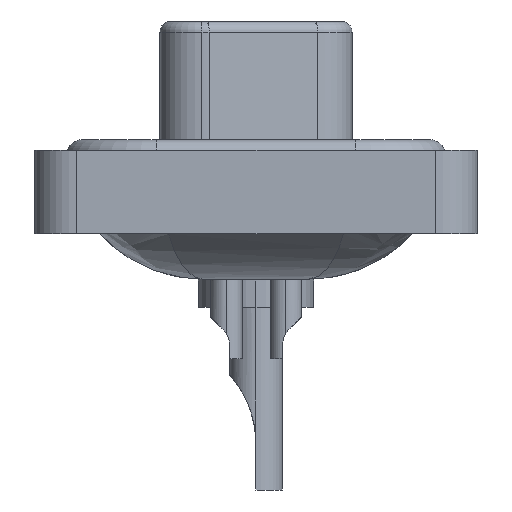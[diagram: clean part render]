
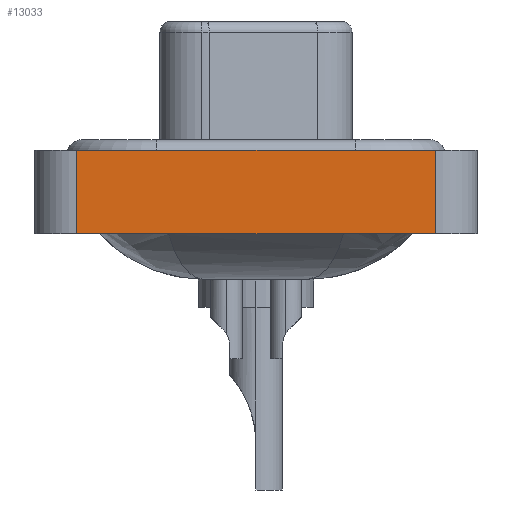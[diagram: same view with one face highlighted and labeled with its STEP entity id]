
A CAD part, left-side view. The second image highlights one B-rep face of the part: STEP entity #13033.
In plain terms, the highlighted planar face has unit normal (-1, 0, 0).
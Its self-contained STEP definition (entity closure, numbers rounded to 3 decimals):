
#166 = EDGE_CURVE ( 'NONE', #8085, #24075, #15353, .T. ) ;
#1186 = CARTESIAN_POINT ( 'NONE',  ( -7.35, 8.55, -3.6 ) ) ;
#1572 = VERTEX_POINT ( 'NONE', #1186 ) ;
#1585 = CARTESIAN_POINT ( 'NONE',  ( -7.35, 8.55, 0.4 ) ) ;
#3384 = DIRECTION ( 'NONE',  ( -1., 0., 0. ) ) ;
#3736 = DIRECTION ( 'NONE',  ( 0., 0., 1. ) ) ;
#4155 = LINE ( 'NONE', #21446, #20333 ) ;
#4780 = LINE ( 'NONE', #17997, #12625 ) ;
#5246 = FACE_OUTER_BOUND ( 'NONE', #16064, .T. ) ;
#5494 = CARTESIAN_POINT ( 'NONE',  ( -7.35, 8.55, -3.6 ) ) ;
#6149 = DIRECTION ( 'NONE',  ( 0., -1., 0. ) ) ;
#6770 = VERTEX_POINT ( 'NONE', #1585 ) ;
#8085 = VERTEX_POINT ( 'NONE', #16706 ) ;
#11334 = VECTOR ( 'NONE', #22654, 1000. ) ;
#11402 = CARTESIAN_POINT ( 'NONE',  ( -7.35, -8.55, -3.6 ) ) ;
#11580 = EDGE_CURVE ( 'NONE', #1572, #6770, #22775, .T. ) ;
#12302 = DIRECTION ( 'NONE',  ( 0., -1., 0. ) ) ;
#12438 = ORIENTED_EDGE ( 'NONE', *, *, #11580, .F. ) ;
#12625 = VECTOR ( 'NONE', #12302, 1000. ) ;
#12902 = DIRECTION ( 'NONE',  ( 0., 0., 1. ) ) ;
#13033 = ADVANCED_FACE ( 'NONE', ( #5246 ), #20309, .T. ) ;
#14110 = EDGE_CURVE ( 'NONE', #6770, #24075, #4780, .T. ) ;
#15353 = LINE ( 'NONE', #11402, #21094 ) ;
#16064 = EDGE_LOOP ( 'NONE', ( #24407, #19536, #12438, #19473 ) ) ;
#16119 = AXIS2_PLACEMENT_3D ( 'NONE', #16842, #3384, #12902 ) ;
#16706 = CARTESIAN_POINT ( 'NONE',  ( -7.35, -8.55, -3.6 ) ) ;
#16842 = CARTESIAN_POINT ( 'NONE',  ( -7.35, -8.55, -3.6 ) ) ;
#17997 = CARTESIAN_POINT ( 'NONE',  ( -7.35, -8.55, 0.4 ) ) ;
#19194 = EDGE_CURVE ( 'NONE', #1572, #8085, #4155, .T. ) ;
#19473 = ORIENTED_EDGE ( 'NONE', *, *, #19194, .T. ) ;
#19536 = ORIENTED_EDGE ( 'NONE', *, *, #14110, .F. ) ;
#20309 = PLANE ( 'NONE',  #16119 ) ;
#20333 = VECTOR ( 'NONE', #6149, 1000. ) ;
#21094 = VECTOR ( 'NONE', #3736, 1000. ) ;
#21097 = CARTESIAN_POINT ( 'NONE',  ( -7.35, -8.55, 0.4 ) ) ;
#21446 = CARTESIAN_POINT ( 'NONE',  ( -7.35, -8.55, -3.6 ) ) ;
#22654 = DIRECTION ( 'NONE',  ( 0., 0., 1. ) ) ;
#22775 = LINE ( 'NONE', #5494, #11334 ) ;
#24075 = VERTEX_POINT ( 'NONE', #21097 ) ;
#24407 = ORIENTED_EDGE ( 'NONE', *, *, #166, .T. ) ;
